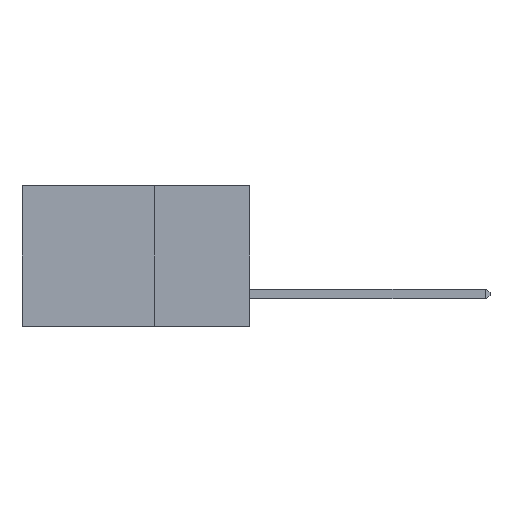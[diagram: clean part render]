
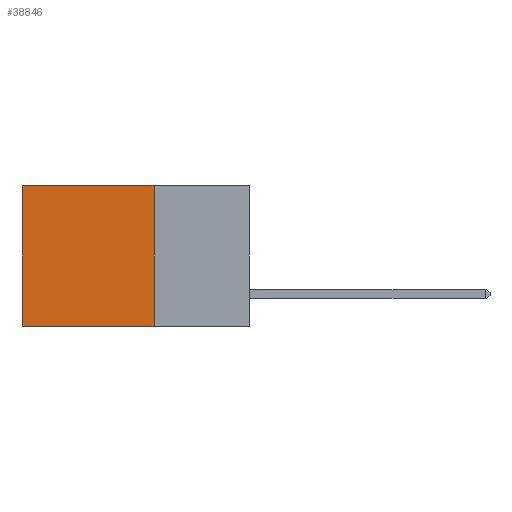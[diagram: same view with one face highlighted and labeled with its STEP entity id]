
A CAD part, left-side view. The second image highlights one B-rep face of the part: STEP entity #38846.
In plain terms, the highlighted planar face has unit normal (-1, 0, 0).
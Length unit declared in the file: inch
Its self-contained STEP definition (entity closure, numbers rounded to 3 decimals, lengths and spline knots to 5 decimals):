
#12 = ORIENTED_EDGE ( 'NONE', *, *, #14464, .F. ) ;
#108 = VECTOR ( 'NONE', #2157, 39.37008 ) ;
#895 = CARTESIAN_POINT ( 'NONE',  ( 0.2875, 0.25, -0.37 ) ) ;
#2157 = DIRECTION ( 'NONE',  ( 0., 0., -1. ) ) ;
#2909 = AXIS2_PLACEMENT_3D ( 'NONE', #37321, #40474, #21769 ) ;
#4293 = EDGE_CURVE ( 'NONE', #40503, #25353, #13099, .T. ) ;
#5377 = CARTESIAN_POINT ( 'NONE',  ( 0.2875, 0.25, 0. ) ) ;
#7506 = CARTESIAN_POINT ( 'NONE',  ( 0.2875, 0.6, 0. ) ) ;
#9056 = EDGE_CURVE ( 'NONE', #25353, #24187, #25055, .T. ) ;
#10755 = DIRECTION ( 'NONE',  ( 0., 0., -1. ) ) ;
#11944 = CARTESIAN_POINT ( 'NONE',  ( 0.2875, 0.25, 0. ) ) ;
#13099 = LINE ( 'NONE', #11944, #18660 ) ;
#14464 = EDGE_CURVE ( 'NONE', #32200, #24187, #39633, .T. ) ;
#15264 = CARTESIAN_POINT ( 'NONE',  ( 0.2875, 0.6, -0.37 ) ) ;
#15466 = PLANE ( 'NONE',  #2909 ) ;
#15745 = VECTOR ( 'NONE', #10755, 39.37008 ) ;
#16751 = EDGE_CURVE ( 'NONE', #40503, #32200, #25437, .T. ) ;
#17161 = ORIENTED_EDGE ( 'NONE', *, *, #9056, .T. ) ;
#18025 = ORIENTED_EDGE ( 'NONE', *, *, #4293, .T. ) ;
#18660 = VECTOR ( 'NONE', #30791, 39.37008 ) ;
#21769 = DIRECTION ( 'NONE',  ( 0., 0., -1. ) ) ;
#24095 = CARTESIAN_POINT ( 'NONE',  ( 0.2875, 0.25, -0.37 ) ) ;
#24187 = VERTEX_POINT ( 'NONE', #15264 ) ;
#25055 = LINE ( 'NONE', #7506, #15745 ) ;
#25353 = VERTEX_POINT ( 'NONE', #39016 ) ;
#25437 = LINE ( 'NONE', #5377, #108 ) ;
#29141 = ORIENTED_EDGE ( 'NONE', *, *, #16751, .F. ) ;
#29248 = CARTESIAN_POINT ( 'NONE',  ( 0.2875, 0.25, 0. ) ) ;
#30339 = FACE_OUTER_BOUND ( 'NONE', #36103, .T. ) ;
#30791 = DIRECTION ( 'NONE',  ( 0., 1., 0. ) ) ;
#31403 = VECTOR ( 'NONE', #39673, 39.37008 ) ;
#32200 = VERTEX_POINT ( 'NONE', #895 ) ;
#36103 = EDGE_LOOP ( 'NONE', ( #17161, #12, #29141, #18025 ) ) ;
#37321 = CARTESIAN_POINT ( 'NONE',  ( 0.2875, 0.25, 0. ) ) ;
#38846 = ADVANCED_FACE ( 'NONE', ( #30339 ), #15466, .F. ) ;
#39016 = CARTESIAN_POINT ( 'NONE',  ( 0.2875, 0.6, 0. ) ) ;
#39633 = LINE ( 'NONE', #24095, #31403 ) ;
#39673 = DIRECTION ( 'NONE',  ( 0., 1., 0. ) ) ;
#40474 = DIRECTION ( 'NONE',  ( 1., 0., 0. ) ) ;
#40503 = VERTEX_POINT ( 'NONE', #29248 ) ;
